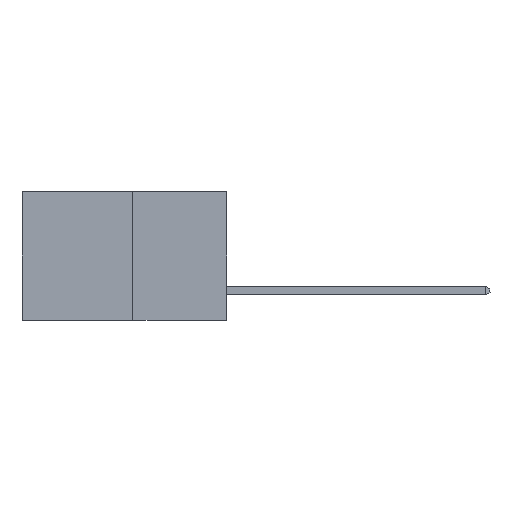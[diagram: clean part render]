
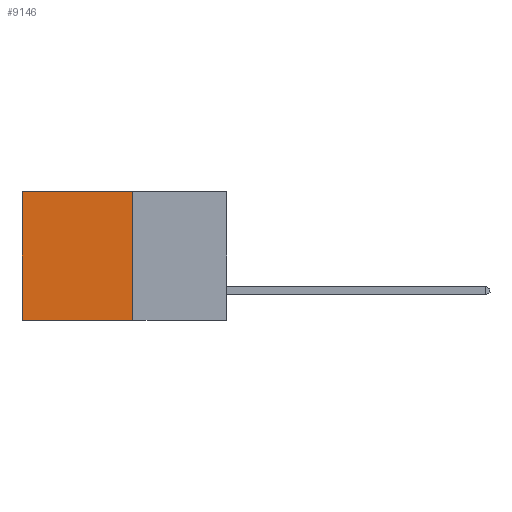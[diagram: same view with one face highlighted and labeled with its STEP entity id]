
A CAD part, left-side view. The second image highlights one B-rep face of the part: STEP entity #9146.
In plain terms, the highlighted planar face has unit normal (-1, 0, 0).
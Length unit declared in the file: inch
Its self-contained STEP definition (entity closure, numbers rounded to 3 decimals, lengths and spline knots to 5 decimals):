
#223 = LINE ( 'NONE', #7364, #4059 ) ;
#297 = DIRECTION ( 'NONE',  ( 0., 0., -1. ) ) ;
#400 = CARTESIAN_POINT ( 'NONE',  ( 0.277, 0.59, -0.37 ) ) ;
#506 = AXIS2_PLACEMENT_3D ( 'NONE', #4113, #4835, #297 ) ;
#689 = DIRECTION ( 'NONE',  ( 0., 0., -1. ) ) ;
#894 = EDGE_LOOP ( 'NONE', ( #3106, #2713, #3585, #4308 ) ) ;
#1332 = LINE ( 'NONE', #6702, #7003 ) ;
#1652 = VERTEX_POINT ( 'NONE', #9387 ) ;
#2369 = EDGE_CURVE ( 'NONE', #9391, #5075, #223, .T. ) ;
#2713 = ORIENTED_EDGE ( 'NONE', *, *, #2369, .F. ) ;
#3106 = ORIENTED_EDGE ( 'NONE', *, *, #7460, .T. ) ;
#3585 = ORIENTED_EDGE ( 'NONE', *, *, #8266, .F. ) ;
#4059 = VECTOR ( 'NONE', #6839, 39.37008 ) ;
#4113 = CARTESIAN_POINT ( 'NONE',  ( 0.277, 0.27, -0.37 ) ) ;
#4308 = ORIENTED_EDGE ( 'NONE', *, *, #8389, .T. ) ;
#4350 = LINE ( 'NONE', #7249, #6237 ) ;
#4517 = CARTESIAN_POINT ( 'NONE',  ( 0.277, 0.59, -0.37 ) ) ;
#4835 = DIRECTION ( 'NONE',  ( 1., 0., 0. ) ) ;
#5075 = VERTEX_POINT ( 'NONE', #400 ) ;
#5833 = DIRECTION ( 'NONE',  ( 0., 0., -1. ) ) ;
#5992 = VERTEX_POINT ( 'NONE', #7413 ) ;
#6237 = VECTOR ( 'NONE', #5833, 39.37008 ) ;
#6432 = FACE_OUTER_BOUND ( 'NONE', #894, .T. ) ;
#6702 = CARTESIAN_POINT ( 'NONE',  ( 0.277, 0.27, 0. ) ) ;
#6839 = DIRECTION ( 'NONE',  ( 0., 1., 0. ) ) ;
#7003 = VECTOR ( 'NONE', #7385, 39.37008 ) ;
#7229 = CARTESIAN_POINT ( 'NONE',  ( 0.277, 0.27, -0.37 ) ) ;
#7249 = CARTESIAN_POINT ( 'NONE',  ( 0.277, 0.27, -0.37 ) ) ;
#7364 = CARTESIAN_POINT ( 'NONE',  ( 0.277, 0.27, -0.37 ) ) ;
#7385 = DIRECTION ( 'NONE',  ( 0., 1., 0. ) ) ;
#7413 = CARTESIAN_POINT ( 'NONE',  ( 0.277, 0.59, 0. ) ) ;
#7460 = EDGE_CURVE ( 'NONE', #5992, #5075, #7937, .T. ) ;
#7937 = LINE ( 'NONE', #4517, #8367 ) ;
#8266 = EDGE_CURVE ( 'NONE', #1652, #9391, #4350, .T. ) ;
#8367 = VECTOR ( 'NONE', #689, 39.37008 ) ;
#8389 = EDGE_CURVE ( 'NONE', #1652, #5992, #1332, .T. ) ;
#8990 = PLANE ( 'NONE',  #506 ) ;
#9146 = ADVANCED_FACE ( 'NONE', ( #6432 ), #8990, .F. ) ;
#9387 = CARTESIAN_POINT ( 'NONE',  ( 0.277, 0.27, 0. ) ) ;
#9391 = VERTEX_POINT ( 'NONE', #7229 ) ;
